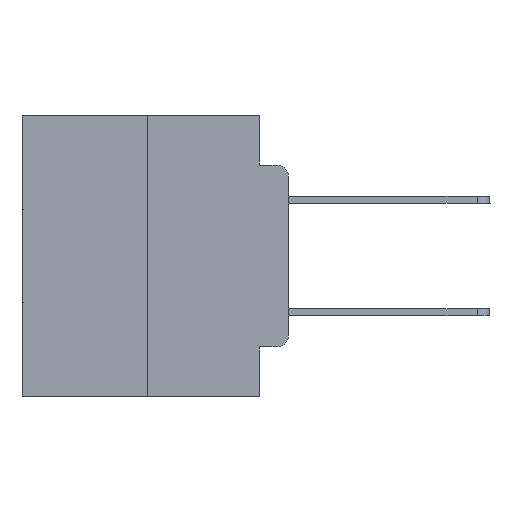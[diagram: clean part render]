
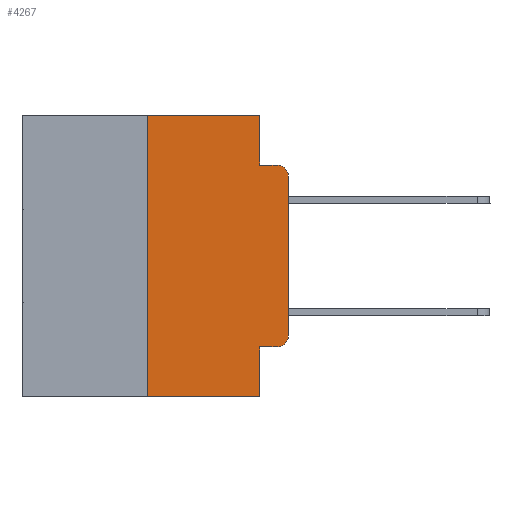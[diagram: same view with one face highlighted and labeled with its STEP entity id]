
A CAD part, left-side view. The second image highlights one B-rep face of the part: STEP entity #4267.
In plain terms, the highlighted planar face has unit normal (-1, 0, 0).
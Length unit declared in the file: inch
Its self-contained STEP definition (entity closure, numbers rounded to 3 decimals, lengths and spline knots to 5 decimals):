
#392 = VERTEX_POINT ( 'NONE', #21765 ) ;
#579 = CARTESIAN_POINT ( 'NONE',  ( 0., 0.051, -0.0885 ) ) ;
#751 = CARTESIAN_POINT ( 'NONE',  ( 0., 0.02, -0.4115 ) ) ;
#945 = CARTESIAN_POINT ( 'NONE',  ( 0., 0.02, -0.1085 ) ) ;
#1066 = DIRECTION ( 'NONE',  ( 1., 0., 0. ) ) ;
#1293 = VERTEX_POINT ( 'NONE', #8642 ) ;
#1350 = EDGE_CURVE ( 'NONE', #1293, #21138, #12837, .T. ) ;
#1503 = CARTESIAN_POINT ( 'NONE',  ( 0., 0.473, 0. ) ) ;
#1881 = DIRECTION ( 'NONE',  ( 0., -1., 0. ) ) ;
#2481 = VECTOR ( 'NONE', #26760, 39.37008 ) ;
#2738 = VECTOR ( 'NONE', #14095, 39.37008 ) ;
#2955 = VERTEX_POINT ( 'NONE', #20890 ) ;
#3148 = VECTOR ( 'NONE', #16645, 39.37008 ) ;
#3230 = DIRECTION ( 'NONE',  ( -1., 0., 0. ) ) ;
#3315 = LINE ( 'NONE', #12133, #3148 ) ;
#3527 = DIRECTION ( 'NONE',  ( 0., 0., -1. ) ) ;
#3563 = CARTESIAN_POINT ( 'NONE',  ( 0., 0., -0.3915 ) ) ;
#3600 = AXIS2_PLACEMENT_3D ( 'NONE', #1503, #1066, #21194 ) ;
#4267 = ADVANCED_FACE ( 'NONE', ( #10337 ), #23481, .F. ) ;
#4432 = DIRECTION ( 'NONE',  ( 0., -1., 0. ) ) ;
#5651 = ORIENTED_EDGE ( 'NONE', *, *, #1350, .T. ) ;
#6126 = EDGE_CURVE ( 'NONE', #22380, #27588, #15996, .T. ) ;
#6298 = VECTOR ( 'NONE', #21433, 39.37008 ) ;
#6745 = AXIS2_PLACEMENT_3D ( 'NONE', #20449, #3230, #12047 ) ;
#7268 = CARTESIAN_POINT ( 'NONE',  ( 0., 0.25, 0. ) ) ;
#8642 = CARTESIAN_POINT ( 'NONE',  ( 0., 0.051, -0.4115 ) ) ;
#9732 = LINE ( 'NONE', #7268, #24525 ) ;
#10285 = EDGE_CURVE ( 'NONE', #11353, #14999, #14928, .T. ) ;
#10337 = FACE_OUTER_BOUND ( 'NONE', #27516, .T. ) ;
#11240 = CARTESIAN_POINT ( 'NONE',  ( 0., 0., -0.1085 ) ) ;
#11353 = VERTEX_POINT ( 'NONE', #11240 ) ;
#11771 = VERTEX_POINT ( 'NONE', #15549 ) ;
#12047 = DIRECTION ( 'NONE',  ( 0., 0., -1. ) ) ;
#12062 = EDGE_CURVE ( 'NONE', #27588, #11771, #20885, .T. ) ;
#12133 = CARTESIAN_POINT ( 'NONE',  ( 0., 0., 0. ) ) ;
#12149 = AXIS2_PLACEMENT_3D ( 'NONE', #945, #13546, #24664 ) ;
#12226 = VECTOR ( 'NONE', #3527, 39.37008 ) ;
#12837 = LINE ( 'NONE', #26423, #15082 ) ;
#12891 = ORIENTED_EDGE ( 'NONE', *, *, #12062, .F. ) ;
#13220 = CARTESIAN_POINT ( 'NONE',  ( 0., 0.25, 0. ) ) ;
#13546 = DIRECTION ( 'NONE',  ( -1., 0., 0. ) ) ;
#14095 = DIRECTION ( 'NONE',  ( 0., -1., 0. ) ) ;
#14928 = CIRCLE ( 'NONE', #12149, 0.02 ) ;
#14999 = VERTEX_POINT ( 'NONE', #27935 ) ;
#15005 = EDGE_CURVE ( 'NONE', #1293, #2955, #19146, .T. ) ;
#15082 = VECTOR ( 'NONE', #4432, 39.37008 ) ;
#15549 = CARTESIAN_POINT ( 'NONE',  ( 0., 0.051, -0.0885 ) ) ;
#15996 = LINE ( 'NONE', #27265, #2738 ) ;
#16645 = DIRECTION ( 'NONE',  ( 0., 0., 1. ) ) ;
#16977 = CARTESIAN_POINT ( 'NONE',  ( 0., 0.051, 0. ) ) ;
#17247 = ORIENTED_EDGE ( 'NONE', *, *, #21508, .F. ) ;
#17511 = CARTESIAN_POINT ( 'NONE',  ( 0., 0.473, -0.5 ) ) ;
#19146 = LINE ( 'NONE', #16977, #6298 ) ;
#19542 = LINE ( 'NONE', #17511, #25796 ) ;
#19621 = CARTESIAN_POINT ( 'NONE',  ( 0., 0.051, 0. ) ) ;
#19637 = ORIENTED_EDGE ( 'NONE', *, *, #27704, .T. ) ;
#19789 = EDGE_CURVE ( 'NONE', #392, #22380, #9732, .T. ) ;
#20449 = CARTESIAN_POINT ( 'NONE',  ( 0., 0.02, -0.3915 ) ) ;
#20885 = LINE ( 'NONE', #23323, #12226 ) ;
#20890 = CARTESIAN_POINT ( 'NONE',  ( 0., 0.051, -0.5 ) ) ;
#21138 = VERTEX_POINT ( 'NONE', #751 ) ;
#21194 = DIRECTION ( 'NONE',  ( 0., 0., -1. ) ) ;
#21287 = ORIENTED_EDGE ( 'NONE', *, *, #15005, .F. ) ;
#21404 = ORIENTED_EDGE ( 'NONE', *, *, #19789, .F. ) ;
#21432 = ORIENTED_EDGE ( 'NONE', *, *, #23581, .T. ) ;
#21433 = DIRECTION ( 'NONE',  ( 0., 0., -1. ) ) ;
#21508 = EDGE_CURVE ( 'NONE', #11771, #14999, #24438, .T. ) ;
#21570 = ORIENTED_EDGE ( 'NONE', *, *, #10285, .T. ) ;
#21765 = CARTESIAN_POINT ( 'NONE',  ( 0., 0.25, -0.5 ) ) ;
#22380 = VERTEX_POINT ( 'NONE', #13220 ) ;
#22896 = CIRCLE ( 'NONE', #6745, 0.02 ) ;
#23004 = ORIENTED_EDGE ( 'NONE', *, *, #6126, .F. ) ;
#23323 = CARTESIAN_POINT ( 'NONE',  ( 0., 0.051, 0. ) ) ;
#23481 = PLANE ( 'NONE',  #3600 ) ;
#23581 = EDGE_CURVE ( 'NONE', #21138, #27640, #22896, .T. ) ;
#24215 = ORIENTED_EDGE ( 'NONE', *, *, #27170, .T. ) ;
#24438 = LINE ( 'NONE', #579, #2481 ) ;
#24525 = VECTOR ( 'NONE', #27361, 39.37008 ) ;
#24664 = DIRECTION ( 'NONE',  ( 0., 0., -1. ) ) ;
#25796 = VECTOR ( 'NONE', #1881, 39.37008 ) ;
#26423 = CARTESIAN_POINT ( 'NONE',  ( 0., 0.051, -0.4115 ) ) ;
#26760 = DIRECTION ( 'NONE',  ( 0., -1., 0. ) ) ;
#27170 = EDGE_CURVE ( 'NONE', #27640, #11353, #3315, .T. ) ;
#27265 = CARTESIAN_POINT ( 'NONE',  ( 0., 0.473, 0. ) ) ;
#27361 = DIRECTION ( 'NONE',  ( 0., 0., 1. ) ) ;
#27516 = EDGE_LOOP ( 'NONE', ( #24215, #21570, #17247, #12891, #23004, #21404, #19637, #21287, #5651, #21432 ) ) ;
#27588 = VERTEX_POINT ( 'NONE', #19621 ) ;
#27640 = VERTEX_POINT ( 'NONE', #3563 ) ;
#27704 = EDGE_CURVE ( 'NONE', #392, #2955, #19542, .T. ) ;
#27935 = CARTESIAN_POINT ( 'NONE',  ( 0., 0.02, -0.0885 ) ) ;
